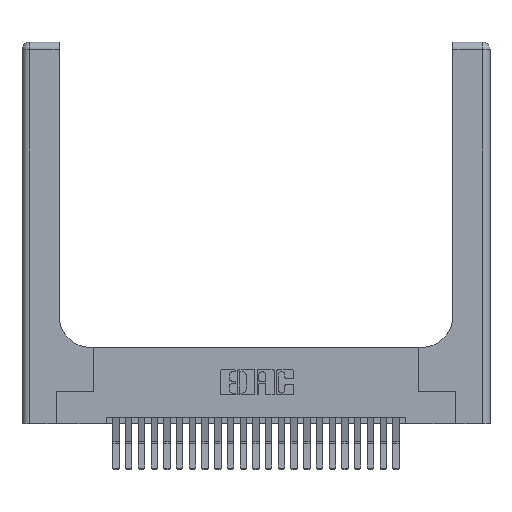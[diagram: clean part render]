
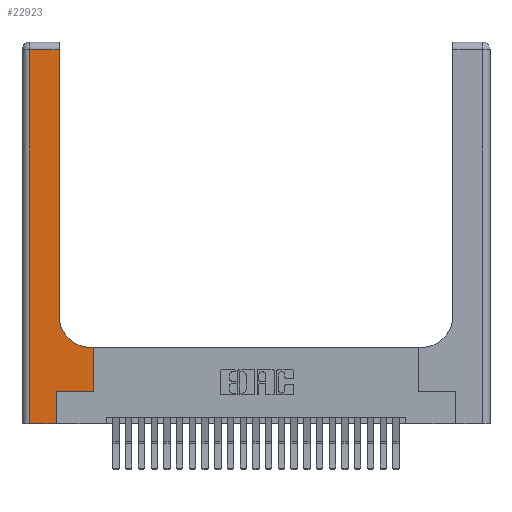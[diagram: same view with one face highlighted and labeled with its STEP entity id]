
A CAD part, top view. The second image highlights one B-rep face of the part: STEP entity #22923.
In plain terms, the highlighted planar face has unit normal (0, 0, 1).
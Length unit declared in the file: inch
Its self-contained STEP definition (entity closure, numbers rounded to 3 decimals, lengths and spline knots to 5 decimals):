
#90 = DIRECTION ( 'NONE',  ( 0., -1., 0. ) ) ;
#245 = VERTEX_POINT ( 'NONE', #4623 ) ;
#771 = CARTESIAN_POINT ( 'NONE',  ( 0.5585, 0.25, 0.37 ) ) ;
#921 = LINE ( 'NONE', #12307, #11748 ) ;
#949 = VECTOR ( 'NONE', #8779, 39.37008 ) ;
#1306 = LINE ( 'NONE', #4958, #11482 ) ;
#1502 = CARTESIAN_POINT ( 'NONE',  ( 0., 2.94, 0.37 ) ) ;
#1854 = EDGE_CURVE ( 'NONE', #18464, #6350, #25301, .T. ) ;
#1928 = VERTEX_POINT ( 'NONE', #25504 ) ;
#2393 = LINE ( 'NONE', #1502, #12601 ) ;
#2631 = VERTEX_POINT ( 'NONE', #4340 ) ;
#3387 = VERTEX_POINT ( 'NONE', #15781 ) ;
#3983 = CARTESIAN_POINT ( 'NONE',  ( 0.06, 2.94, 0.37 ) ) ;
#4118 = VECTOR ( 'NONE', #23292, 39.37008 ) ;
#4340 = CARTESIAN_POINT ( 'NONE',  ( 0.269, 0., 0.37 ) ) ;
#4467 = EDGE_CURVE ( 'NONE', #245, #22101, #17654, .T. ) ;
#4623 = CARTESIAN_POINT ( 'NONE',  ( 0.269, 0.25, 0.37 ) ) ;
#4958 = CARTESIAN_POINT ( 'NONE',  ( 0.2915, 3., 0.37 ) ) ;
#5046 = AXIS2_PLACEMENT_3D ( 'NONE', #17354, #19401, #7464 ) ;
#5064 = ORIENTED_EDGE ( 'NONE', *, *, #19159, .T. ) ;
#5402 = PLANE ( 'NONE',  #5046 ) ;
#6350 = VERTEX_POINT ( 'NONE', #10290 ) ;
#6920 = ORIENTED_EDGE ( 'NONE', *, *, #4467, .T. ) ;
#7022 = DIRECTION ( 'NONE',  ( 0., 1., 0. ) ) ;
#7254 = FACE_OUTER_BOUND ( 'NONE', #24983, .T. ) ;
#7437 = EDGE_CURVE ( 'NONE', #10094, #10422, #2393, .T. ) ;
#7464 = DIRECTION ( 'NONE',  ( -1., 0., 0. ) ) ;
#7588 = EDGE_CURVE ( 'NONE', #3387, #2631, #14182, .T. ) ;
#8120 = ORIENTED_EDGE ( 'NONE', *, *, #19195, .T. ) ;
#8727 = CARTESIAN_POINT ( 'NONE',  ( 0.5585, 0.6, 0.37 ) ) ;
#8779 = DIRECTION ( 'NONE',  ( 0., 1., 0. ) ) ;
#8914 = LINE ( 'NONE', #11850, #14930 ) ;
#8952 = CARTESIAN_POINT ( 'NONE',  ( 0.5415, 0.85, 0.37 ) ) ;
#9038 = DIRECTION ( 'NONE',  ( 1., 0., 0. ) ) ;
#10094 = VERTEX_POINT ( 'NONE', #24551 ) ;
#10209 = ORIENTED_EDGE ( 'NONE', *, *, #19602, .T. ) ;
#10290 = CARTESIAN_POINT ( 'NONE',  ( 0.5415, 0.6, 0.37 ) ) ;
#10422 = VERTEX_POINT ( 'NONE', #3983 ) ;
#10986 = DIRECTION ( 'NONE',  ( 1., 0., 0. ) ) ;
#11482 = VECTOR ( 'NONE', #7022, 39.37008 ) ;
#11748 = VECTOR ( 'NONE', #90, 39.37008 ) ;
#11850 = CARTESIAN_POINT ( 'NONE',  ( 0.269, 0., 0.37 ) ) ;
#11895 = AXIS2_PLACEMENT_3D ( 'NONE', #8952, #22837, #10986 ) ;
#12164 = CARTESIAN_POINT ( 'NONE',  ( 0., 0., 0.37 ) ) ;
#12307 = CARTESIAN_POINT ( 'NONE',  ( 0.06, 3., 0.37 ) ) ;
#12381 = VECTOR ( 'NONE', #9038, 39.37008 ) ;
#12601 = VECTOR ( 'NONE', #13465, 39.37008 ) ;
#13465 = DIRECTION ( 'NONE',  ( -1., 0., 0. ) ) ;
#14182 = LINE ( 'NONE', #12164, #20597 ) ;
#14930 = VECTOR ( 'NONE', #23672, 39.37008 ) ;
#15049 = CARTESIAN_POINT ( 'NONE',  ( 0.269, 0.25, 0.37 ) ) ;
#15580 = EDGE_CURVE ( 'NONE', #1928, #10094, #1306, .T. ) ;
#15781 = CARTESIAN_POINT ( 'NONE',  ( 0.06, 0., 0.37 ) ) ;
#15866 = LINE ( 'NONE', #22663, #949 ) ;
#16786 = ORIENTED_EDGE ( 'NONE', *, *, #1854, .T. ) ;
#17067 = ORIENTED_EDGE ( 'NONE', *, *, #19495, .T. ) ;
#17354 = CARTESIAN_POINT ( 'NONE',  ( 0., 3., 0.37 ) ) ;
#17654 = LINE ( 'NONE', #15049, #12381 ) ;
#18464 = VERTEX_POINT ( 'NONE', #8727 ) ;
#18483 = ORIENTED_EDGE ( 'NONE', *, *, #7437, .T. ) ;
#19159 = EDGE_CURVE ( 'NONE', #22101, #18464, #15866, .T. ) ;
#19161 = DIRECTION ( 'NONE',  ( 1., 0., 0. ) ) ;
#19195 = EDGE_CURVE ( 'NONE', #6350, #1928, #25039, .T. ) ;
#19401 = DIRECTION ( 'NONE',  ( 0., 0., -1. ) ) ;
#19434 = CARTESIAN_POINT ( 'NONE',  ( 0.2915, 0.6, 0.37 ) ) ;
#19495 = EDGE_CURVE ( 'NONE', #2631, #245, #8914, .T. ) ;
#19602 = EDGE_CURVE ( 'NONE', #10422, #3387, #921, .T. ) ;
#20597 = VECTOR ( 'NONE', #19161, 39.37008 ) ;
#22101 = VERTEX_POINT ( 'NONE', #771 ) ;
#22663 = CARTESIAN_POINT ( 'NONE',  ( 0.5585, 0.25, 0.37 ) ) ;
#22837 = DIRECTION ( 'NONE',  ( 0., 0., -1. ) ) ;
#22923 = ADVANCED_FACE ( 'NONE', ( #7254 ), #5402, .F. ) ;
#23292 = DIRECTION ( 'NONE',  ( -1., 0., 0. ) ) ;
#23672 = DIRECTION ( 'NONE',  ( 0., 1., 0. ) ) ;
#23823 = ORIENTED_EDGE ( 'NONE', *, *, #7588, .T. ) ;
#24027 = ORIENTED_EDGE ( 'NONE', *, *, #15580, .T. ) ;
#24551 = CARTESIAN_POINT ( 'NONE',  ( 0.2915, 2.94, 0.37 ) ) ;
#24983 = EDGE_LOOP ( 'NONE', ( #24027, #18483, #10209, #23823, #17067, #6920, #5064, #16786, #8120 ) ) ;
#25039 = CIRCLE ( 'NONE', #11895, 0.25 ) ;
#25301 = LINE ( 'NONE', #19434, #4118 ) ;
#25504 = CARTESIAN_POINT ( 'NONE',  ( 0.2915, 0.85, 0.37 ) ) ;
